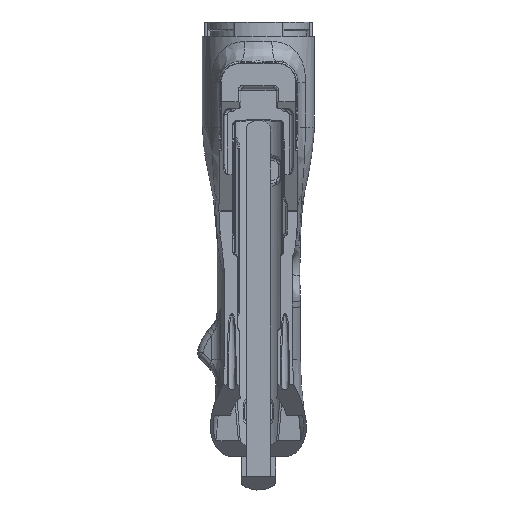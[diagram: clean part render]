
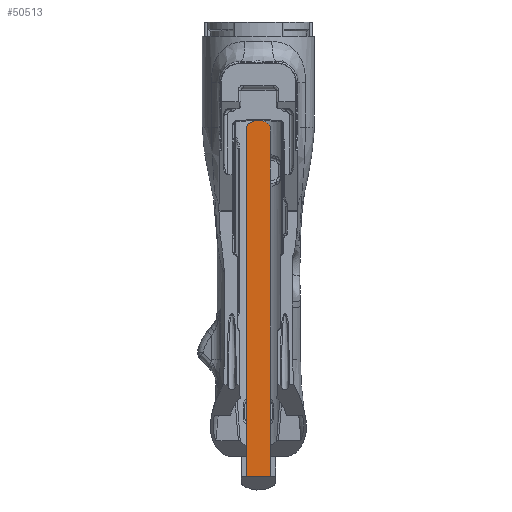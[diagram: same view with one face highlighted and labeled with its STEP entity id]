
A CAD part, front view. The second image highlights one B-rep face of the part: STEP entity #50513.
In plain terms, the highlighted planar face has unit normal (0, -1, 0).
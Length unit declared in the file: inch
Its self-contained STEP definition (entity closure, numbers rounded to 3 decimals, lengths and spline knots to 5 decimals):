
#1164 = DIRECTION ( 'NONE',  ( 0., 0., 1. ) ) ;
#1607 = EDGE_CURVE ( 'NONE', #38101, #46480, #46690, .T. ) ;
#2220 = CARTESIAN_POINT ( 'NONE',  ( -0.215, 1.02, -6.65 ) ) ;
#4321 = LINE ( 'NONE', #24619, #6141 ) ;
#6141 = VECTOR ( 'NONE', #14799, 39.37008 ) ;
#8158 = LINE ( 'NONE', #37597, #41089 ) ;
#8476 = DIRECTION ( 'NONE',  ( 1., 0., 0. ) ) ;
#9805 = DIRECTION ( 'NONE',  ( 0., 1., 0. ) ) ;
#10542 = EDGE_CURVE ( 'NONE', #42561, #16609, #4321, .T. ) ;
#12035 = CARTESIAN_POINT ( 'NONE',  ( 0.215, 1.02, -6.36576 ) ) ;
#14620 = VECTOR ( 'NONE', #26774, 39.37008 ) ;
#14799 = DIRECTION ( 'NONE',  ( 0., 0., -1. ) ) ;
#15042 = CARTESIAN_POINT ( 'NONE',  ( 0., 1.02, -0.25 ) ) ;
#16609 = VERTEX_POINT ( 'NONE', #12035 ) ;
#17475 = EDGE_CURVE ( 'NONE', #38101, #16609, #8158, .T. ) ;
#19872 = EDGE_LOOP ( 'NONE', ( #48755, #57028, #33043, #57138 ) ) ;
#23591 = PLANE ( 'NONE',  #51655 ) ;
#24619 = CARTESIAN_POINT ( 'NONE',  ( 0.215, 1.02, -0.12243 ) ) ;
#26028 = DIRECTION ( 'NONE',  ( 0., 1., 0. ) ) ;
#26774 = DIRECTION ( 'NONE',  ( 0., 0., 1. ) ) ;
#33043 = ORIENTED_EDGE ( 'NONE', *, *, #10542, .F. ) ;
#35821 = CARTESIAN_POINT ( 'NONE',  ( 0., 1.02, -0.25 ) ) ;
#36484 = CARTESIAN_POINT ( 'NONE',  ( -0.215, 1.02, -0.12243 ) ) ;
#37597 = CARTESIAN_POINT ( 'NONE',  ( 0., 1.02, -6.36576 ) ) ;
#38101 = VERTEX_POINT ( 'NONE', #41723 ) ;
#39872 = DIRECTION ( 'NONE',  ( 0., 0., 1. ) ) ;
#41089 = VECTOR ( 'NONE', #8476, 39.37008 ) ;
#41723 = CARTESIAN_POINT ( 'NONE',  ( -0.215, 1.02, -6.36576 ) ) ;
#42561 = VERTEX_POINT ( 'NONE', #49912 ) ;
#46480 = VERTEX_POINT ( 'NONE', #36484 ) ;
#46496 = EDGE_CURVE ( 'NONE', #46480, #42561, #51968, .T. ) ;
#46690 = LINE ( 'NONE', #2220, #14620 ) ;
#48755 = ORIENTED_EDGE ( 'NONE', *, *, #1607, .F. ) ;
#49912 = CARTESIAN_POINT ( 'NONE',  ( 0.215, 1.02, -0.12243 ) ) ;
#50513 = ADVANCED_FACE ( 'NONE', ( #58225 ), #23591, .F. ) ;
#51655 = AXIS2_PLACEMENT_3D ( 'NONE', #15042, #9805, #39872 ) ;
#51968 = CIRCLE ( 'NONE', #56116, 0.25 ) ;
#56116 = AXIS2_PLACEMENT_3D ( 'NONE', #35821, #26028, #1164 ) ;
#57028 = ORIENTED_EDGE ( 'NONE', *, *, #17475, .T. ) ;
#57138 = ORIENTED_EDGE ( 'NONE', *, *, #46496, .F. ) ;
#58225 = FACE_OUTER_BOUND ( 'NONE', #19872, .T. ) ;
